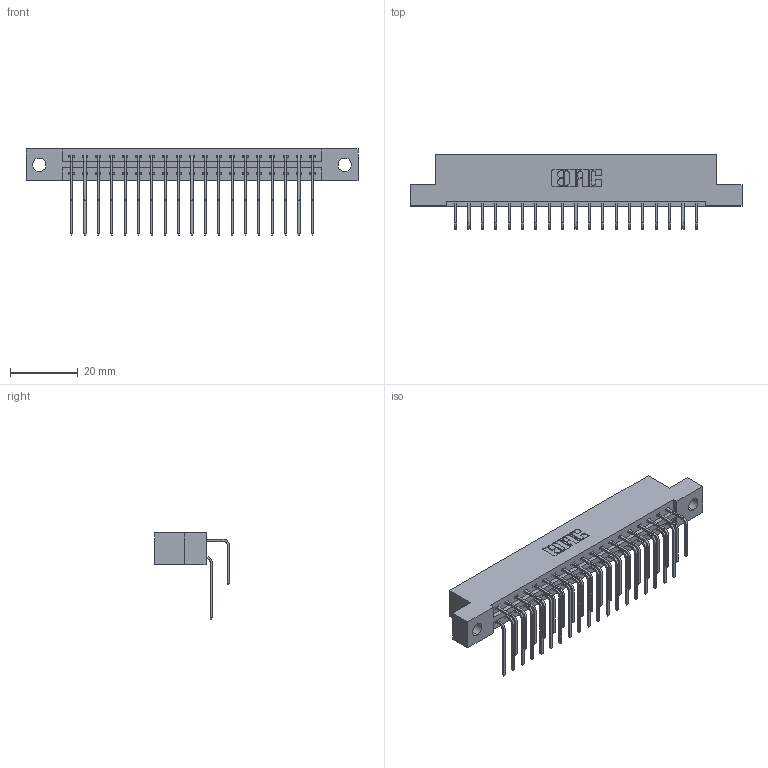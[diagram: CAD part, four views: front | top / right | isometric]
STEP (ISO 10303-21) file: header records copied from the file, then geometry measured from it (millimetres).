
FILE_DESCRIPTION (( 'STEP AP203' ), '1' );
FILE_NAME ('387-038-558-204.STEP', '2019-10-17T22:22:19', ( '' ), ( '' ), 'SwSTEP 2.0', 'SolidWorks 2016', '' );
FILE_SCHEMA (( 'CONFIG_CONTROL_DESIGN' ));
Length unit declared in the file: inch
Products named in the file (4): 345-292-001_558 559 Tail - 1; 345-292-001_558 Tail - 2; 387-038-558-204; 337 Part_Flush Mounting Lugs - 0.156 Dia-TH
Assembly tree (39 placements, depth 2):
  387-038-558-204
    337 Part_Flush Mounting Lugs - 0.156 Dia-TH
    345-292-001_558 559 Tail - 1  x19
    345-292-001_558 Tail - 2  x19
Bounding box: 98.3 x 22.17 x 25.53 mm (x, y, z)
Volume: 10184.6 mm3; surface area: 12188.4 mm2
Topology: 39 solids, 39 shells, 2242 faces, 6657 edges, 4386 vertices
Faces by surface type: plane 1590, cylinder 652
Entity records: 19493 total; most frequent: CARTESIAN_POINT 3349, ORIENTED_EDGE 3234, DIRECTION 2873, EDGE_CURVE 1617, VECTOR 1449, LINE 1449, VERTEX_POINT 1074, AXIS2_PLACEMENT_3D 712
